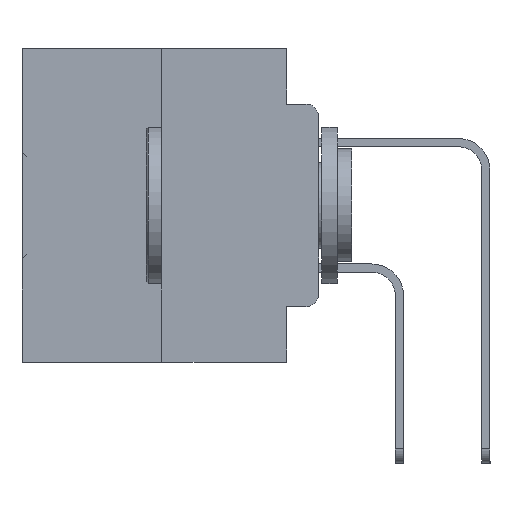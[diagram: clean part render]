
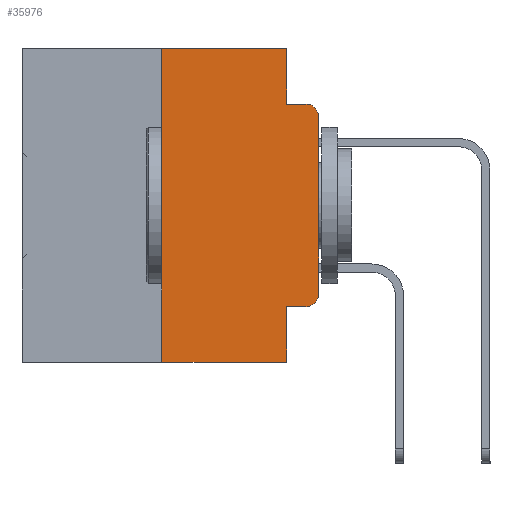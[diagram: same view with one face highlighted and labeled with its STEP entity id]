
A CAD part, left-side view. The second image highlights one B-rep face of the part: STEP entity #35976.
In plain terms, the highlighted planar face has unit normal (-1, 0, 0).
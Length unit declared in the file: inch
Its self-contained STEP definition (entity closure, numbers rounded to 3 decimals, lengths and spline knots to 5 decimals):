
#459 = CARTESIAN_POINT ( 'NONE',  ( 0., 0.02, -0.4115 ) ) ;
#547 = CARTESIAN_POINT ( 'NONE',  ( 0., 0., -0.1085 ) ) ;
#758 = EDGE_CURVE ( 'NONE', #11536, #23041, #10160, .T. ) ;
#1172 = CARTESIAN_POINT ( 'NONE',  ( 0., 0.051, -0.4115 ) ) ;
#1205 = AXIS2_PLACEMENT_3D ( 'NONE', #30595, #13883, #33312 ) ;
#1210 = EDGE_CURVE ( 'NONE', #17005, #20318, #9225, .T. ) ;
#2057 = VECTOR ( 'NONE', #18219, 39.37008 ) ;
#2231 = VERTEX_POINT ( 'NONE', #30173 ) ;
#3124 = VECTOR ( 'NONE', #6952, 39.37008 ) ;
#3335 = EDGE_CURVE ( 'NONE', #20992, #21218, #6370, .T. ) ;
#3616 = EDGE_CURVE ( 'NONE', #20318, #23041, #28509, .T. ) ;
#4536 = EDGE_CURVE ( 'NONE', #2231, #20992, #10818, .T. ) ;
#5000 = VECTOR ( 'NONE', #13831, 39.37008 ) ;
#5691 = VECTOR ( 'NONE', #16102, 39.37008 ) ;
#6370 = CIRCLE ( 'NONE', #9825, 0.02 ) ;
#6952 = DIRECTION ( 'NONE',  ( 0., -1., 0. ) ) ;
#7115 = EDGE_CURVE ( 'NONE', #12738, #21092, #12483, .T. ) ;
#8084 = ORIENTED_EDGE ( 'NONE', *, *, #30179, .T. ) ;
#8101 = PLANE ( 'NONE',  #1205 ) ;
#8196 = ORIENTED_EDGE ( 'NONE', *, *, #758, .T. ) ;
#8626 = ORIENTED_EDGE ( 'NONE', *, *, #3616, .F. ) ;
#8797 = ORIENTED_EDGE ( 'NONE', *, *, #1210, .F. ) ;
#9055 = ORIENTED_EDGE ( 'NONE', *, *, #18293, .F. ) ;
#9090 = DIRECTION ( 'NONE',  ( 0., 0., 1. ) ) ;
#9225 = LINE ( 'NONE', #16544, #2057 ) ;
#9453 = ORIENTED_EDGE ( 'NONE', *, *, #7115, .F. ) ;
#9590 = ORIENTED_EDGE ( 'NONE', *, *, #32932, .T. ) ;
#9779 = AXIS2_PLACEMENT_3D ( 'NONE', #33047, #31876, #30927 ) ;
#9825 = AXIS2_PLACEMENT_3D ( 'NONE', #12600, #32101, #15474 ) ;
#9912 = ORIENTED_EDGE ( 'NONE', *, *, #29227, .F. ) ;
#10160 = CIRCLE ( 'NONE', #9779, 0.02 ) ;
#10162 = ORIENTED_EDGE ( 'NONE', *, *, #4536, .T. ) ;
#10451 = ORIENTED_EDGE ( 'NONE', *, *, #3335, .T. ) ;
#10818 = LINE ( 'NONE', #1172, #3124 ) ;
#11536 = VERTEX_POINT ( 'NONE', #547 ) ;
#12483 = LINE ( 'NONE', #24438, #5691 ) ;
#12580 = CARTESIAN_POINT ( 'NONE',  ( 0., 0.25, 0. ) ) ;
#12600 = CARTESIAN_POINT ( 'NONE',  ( 0., 0.02, -0.3915 ) ) ;
#12738 = VERTEX_POINT ( 'NONE', #34646 ) ;
#13831 = DIRECTION ( 'NONE',  ( 0., -1., 0. ) ) ;
#13883 = DIRECTION ( 'NONE',  ( 1., 0., 0. ) ) ;
#15474 = DIRECTION ( 'NONE',  ( 0., 0., -1. ) ) ;
#15689 = CARTESIAN_POINT ( 'NONE',  ( 0., 0.051, 0. ) ) ;
#16102 = DIRECTION ( 'NONE',  ( 0., 0., 1. ) ) ;
#16544 = CARTESIAN_POINT ( 'NONE',  ( 0., 0.051, 0. ) ) ;
#16575 = CARTESIAN_POINT ( 'NONE',  ( 0., 0.051, -0.0885 ) ) ;
#17005 = VERTEX_POINT ( 'NONE', #15689 ) ;
#17710 = CARTESIAN_POINT ( 'NONE',  ( 0., 0., 0. ) ) ;
#17753 = DIRECTION ( 'NONE',  ( 0., -1., 0. ) ) ;
#18219 = DIRECTION ( 'NONE',  ( 0., 0., -1. ) ) ;
#18293 = EDGE_CURVE ( 'NONE', #21092, #17005, #31181, .T. ) ;
#18922 = LINE ( 'NONE', #34264, #32735 ) ;
#19144 = DIRECTION ( 'NONE',  ( 0., 0., -1. ) ) ;
#20318 = VERTEX_POINT ( 'NONE', #26979 ) ;
#20355 = DIRECTION ( 'NONE',  ( 0., -1., 0. ) ) ;
#20992 = VERTEX_POINT ( 'NONE', #459 ) ;
#21092 = VERTEX_POINT ( 'NONE', #12580 ) ;
#21218 = VERTEX_POINT ( 'NONE', #32431 ) ;
#22512 = VECTOR ( 'NONE', #9090, 39.37008 ) ;
#23041 = VERTEX_POINT ( 'NONE', #24531 ) ;
#23880 = VECTOR ( 'NONE', #20355, 39.37008 ) ;
#24438 = CARTESIAN_POINT ( 'NONE',  ( 0., 0.25, 0. ) ) ;
#24531 = CARTESIAN_POINT ( 'NONE',  ( 0., 0.02, -0.0885 ) ) ;
#25207 = LINE ( 'NONE', #35580, #26083 ) ;
#25877 = CARTESIAN_POINT ( 'NONE',  ( 0., 0.473, 0. ) ) ;
#26083 = VECTOR ( 'NONE', #19144, 39.37008 ) ;
#26979 = CARTESIAN_POINT ( 'NONE',  ( 0., 0.051, -0.0885 ) ) ;
#28509 = LINE ( 'NONE', #16575, #5000 ) ;
#28520 = CARTESIAN_POINT ( 'NONE',  ( 0., 0.051, -0.5 ) ) ;
#28996 = LINE ( 'NONE', #17710, #22512 ) ;
#29227 = EDGE_CURVE ( 'NONE', #2231, #30742, #25207, .T. ) ;
#30173 = CARTESIAN_POINT ( 'NONE',  ( 0., 0.051, -0.4115 ) ) ;
#30179 = EDGE_CURVE ( 'NONE', #21218, #11536, #28996, .T. ) ;
#30595 = CARTESIAN_POINT ( 'NONE',  ( 0., 0.473, 0. ) ) ;
#30742 = VERTEX_POINT ( 'NONE', #28520 ) ;
#30927 = DIRECTION ( 'NONE',  ( 0., 0., -1. ) ) ;
#31077 = EDGE_LOOP ( 'NONE', ( #8084, #8196, #8626, #8797, #9055, #9453, #9590, #9912, #10162, #10451 ) ) ;
#31181 = LINE ( 'NONE', #25877, #23880 ) ;
#31876 = DIRECTION ( 'NONE',  ( -1., 0., 0. ) ) ;
#32101 = DIRECTION ( 'NONE',  ( -1., 0., 0. ) ) ;
#32431 = CARTESIAN_POINT ( 'NONE',  ( 0., 0., -0.3915 ) ) ;
#32735 = VECTOR ( 'NONE', #17753, 39.37008 ) ;
#32932 = EDGE_CURVE ( 'NONE', #12738, #30742, #18922, .T. ) ;
#33047 = CARTESIAN_POINT ( 'NONE',  ( 0., 0.02, -0.1085 ) ) ;
#33312 = DIRECTION ( 'NONE',  ( 0., 0., -1. ) ) ;
#34264 = CARTESIAN_POINT ( 'NONE',  ( 0., 0.473, -0.5 ) ) ;
#34646 = CARTESIAN_POINT ( 'NONE',  ( 0., 0.25, -0.5 ) ) ;
#35506 = FACE_OUTER_BOUND ( 'NONE', #31077, .T. ) ;
#35580 = CARTESIAN_POINT ( 'NONE',  ( 0., 0.051, 0. ) ) ;
#35976 = ADVANCED_FACE ( 'NONE', ( #35506 ), #8101, .F. ) ;
